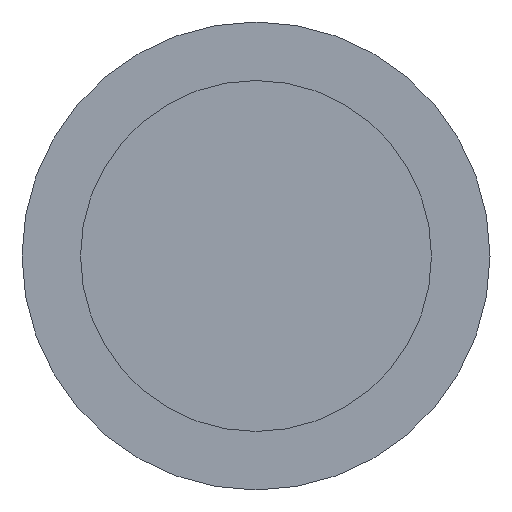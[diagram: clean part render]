
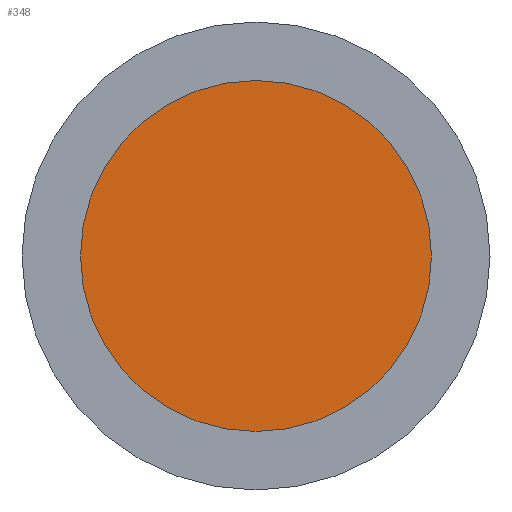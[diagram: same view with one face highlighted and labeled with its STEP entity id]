
A CAD part, front view. The second image highlights one B-rep face of the part: STEP entity #348.
In plain terms, the highlighted planar face has unit normal (0, -1, 0).
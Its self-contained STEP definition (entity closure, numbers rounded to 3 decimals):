
#21 = DIRECTION ( 'NONE',  ( 1., 0., 0. ) ) ;
#22 = DIRECTION ( 'NONE',  ( 0., 1., 0. ) ) ;
#23 = CARTESIAN_POINT ( 'NONE',  ( 0., -9.817, 0. ) ) ;
#62 = DIRECTION ( 'NONE',  ( 0., 0., -1. ) ) ;
#63 = DIRECTION ( 'NONE',  ( 0., -1., 0. ) ) ;
#66 = CARTESIAN_POINT ( 'NONE',  ( -1.238, -9.817, 0. ) ) ;
#67 = PLANE ( 'NONE',  #279 ) ;
#84 = CIRCLE ( 'NONE', #291, 1.238 ) ;
#86 = DIRECTION ( 'NONE',  ( 1., 0., 0. ) ) ;
#87 = DIRECTION ( 'NONE',  ( 0., 1., 0. ) ) ;
#88 = CARTESIAN_POINT ( 'NONE',  ( 0., -9.817, 0. ) ) ;
#147 = CARTESIAN_POINT ( 'NONE',  ( 1.238, -9.817, 0. ) ) ;
#154 = CARTESIAN_POINT ( 'NONE',  ( -1.238, -9.817, 0. ) ) ;
#162 = ORIENTED_EDGE ( 'NONE', *, *, #341, .F. ) ;
#173 = EDGE_LOOP ( 'NONE', ( #162, #250 ) ) ;
#190 = CIRCLE ( 'NONE', #269, 1.238 ) ;
#227 = VERTEX_POINT ( 'NONE', #154 ) ;
#250 = ORIENTED_EDGE ( 'NONE', *, *, #364, .F. ) ;
#269 = AXIS2_PLACEMENT_3D ( 'NONE', #23, #22, #21 ) ;
#278 = VERTEX_POINT ( 'NONE', #147 ) ;
#279 = AXIS2_PLACEMENT_3D ( 'NONE', #66, #63, #62 ) ;
#291 = AXIS2_PLACEMENT_3D ( 'NONE', #88, #87, #86 ) ;
#341 = EDGE_CURVE ( 'NONE', #227, #278, #84, .T. ) ;
#348 = ADVANCED_FACE ( 'NONE', ( #384 ), #67, .T. ) ;
#364 = EDGE_CURVE ( 'NONE', #278, #227, #190, .T. ) ;
#384 = FACE_OUTER_BOUND ( 'NONE', #173, .T. ) ;
